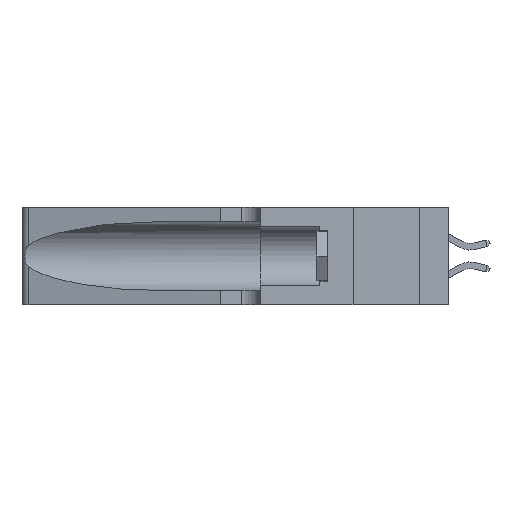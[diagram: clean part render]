
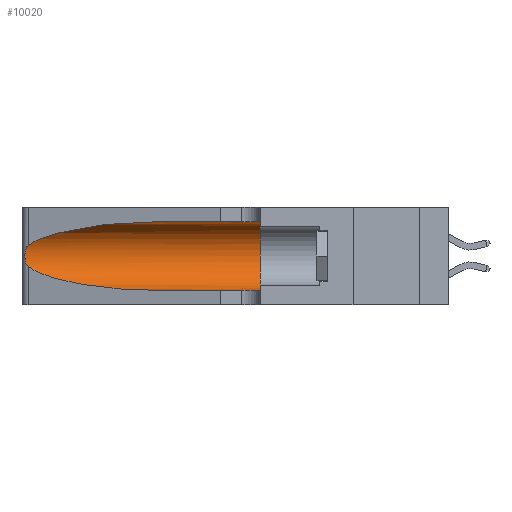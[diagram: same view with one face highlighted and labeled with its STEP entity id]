
A CAD part, left-side view. The second image highlights one B-rep face of the part: STEP entity #10020.
In plain terms, the highlighted cylindrical face has radius 3.308 mm (diameter 6.617 mm), a partial arc.
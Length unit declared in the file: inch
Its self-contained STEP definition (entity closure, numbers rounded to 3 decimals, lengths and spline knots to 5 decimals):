
#9 = CARTESIAN_POINT ( 'NONE',  ( 0.18966, 0.96281, 0.05475 ) ) ;
#45 = CARTESIAN_POINT ( 'NONE',  ( 0.25555, 1.22994, 0.2215 ) ) ;
#142 = LINE ( 'NONE', #4541, #23501 ) ;
#310 = CARTESIAN_POINT ( 'NONE',  ( 0.25555, 1.22993, 0.14849 ) ) ;
#469 = DIRECTION ( 'NONE',  ( 0., 0., 1. ) ) ;
#746 = EDGE_CURVE ( 'NONE', #12465, #10839, #22938, .T. ) ;
#1128 = DIRECTION ( 'NONE',  ( 0., -1., 0. ) ) ;
#1130 = DIRECTION ( 'NONE',  ( 0., -1., 0. ) ) ;
#1212 = DIRECTION ( 'NONE',  ( 0., 0., -1. ) ) ;
#1377 = CARTESIAN_POINT ( 'NONE',  ( 0.1305, 1.61858, 0.185 ) ) ;
#2003 = CARTESIAN_POINT ( 'NONE',  ( 0.26017, 1.23833, 0.17102 ) ) ;
#3063 = B_SPLINE_CURVE_WITH_KNOTS ( 'NONE', 3,
 ( #4125, #45, #13833, #4030, #6064, #17570, #15807, #13556, #2003, #5970, #15544, #9962, #310, #23531 ),
 .UNSPECIFIED., .F., .F.,
 ( 4, 2, 2, 2, 2, 2, 4 ),
 ( 0., 0.00027, 0.00053, 0.00107, 0.0016, 0.00187, 0.00214 ),
 .UNSPECIFIED. ) ;
#4030 = CARTESIAN_POINT ( 'NONE',  ( 0.25787, 1.23484, 0.2124 ) ) ;
#4125 = CARTESIAN_POINT ( 'NONE',  ( 0.25487, 1.22718, 0.22369 ) ) ;
#4434 = CARTESIAN_POINT ( 'NONE',  ( 0.1305, 0.35, 0.31525 ) ) ;
#4541 = CARTESIAN_POINT ( 'NONE',  ( 0.1305, 1.61858, 0.31525 ) ) ;
#4695 = LINE ( 'NONE', #10105, #17401 ) ;
#4782 = CYLINDRICAL_SURFACE ( 'NONE', #9889, 0.13025 ) ;
#4849 = CARTESIAN_POINT ( 'NONE',  ( 0.2373, 1.15595, 0.28018 ) ) ;
#5970 = CARTESIAN_POINT ( 'NONE',  ( 0.25856, 1.23593, 0.16098 ) ) ;
#6030 = CARTESIAN_POINT ( 'NONE',  ( 0.1305, 0.72297, 0.05475 ) ) ;
#6064 = CARTESIAN_POINT ( 'NONE',  ( 0.25854, 1.2359, 0.20912 ) ) ;
#6869 = EDGE_CURVE ( 'NONE', #24837, #12465, #3063, .T. ) ;
#6911 = ORIENTED_EDGE ( 'NONE', *, *, #746, .T. ) ;
#7009 = VERTEX_POINT ( 'NONE', #23465 ) ;
#7411 = VERTEX_POINT ( 'NONE', #11786 ) ;
#9354 = CIRCLE ( 'NONE', #14118, 0.13025 ) ;
#9669 = CARTESIAN_POINT ( 'NONE',  ( 0.2373, 1.15595, 0.08982 ) ) ;
#9889 = AXIS2_PLACEMENT_3D ( 'NONE', #1377, #1128, #1212 ) ;
#9962 = CARTESIAN_POINT ( 'NONE',  ( 0.25639, 1.23186, 0.15144 ) ) ;
#10020 = ADVANCED_FACE ( 'NONE', ( #11404 ), #4782, .F. ) ;
#10105 = CARTESIAN_POINT ( 'NONE',  ( 0.1305, 1.61858, 0.05475 ) ) ;
#10591 = CARTESIAN_POINT ( 'NONE',  ( 0.1305, 0.72297, 0.31525 ) ) ;
#10839 = VERTEX_POINT ( 'NONE', #24407 ) ;
#11404 = FACE_OUTER_BOUND ( 'NONE', #14740, .T. ) ;
#11680 = CARTESIAN_POINT ( 'NONE',  ( 0.25487, 1.22718, 0.14631 ) ) ;
#11786 = CARTESIAN_POINT ( 'NONE',  ( 0.1305, 0.72297, 0.31525 ) ) ;
#12046 = DIRECTION ( 'NONE',  ( 0., 1., 0. ) ) ;
#12465 = VERTEX_POINT ( 'NONE', #20478 ) ;
#12801 = ORIENTED_EDGE ( 'NONE', *, *, #19139, .F. ) ;
#12835 = EDGE_CURVE ( 'NONE', #21500, #7009, #9354, .T. ) ;
#13535 = CARTESIAN_POINT ( 'NONE',  ( 0.25487, 1.22718, 0.22369 ) ) ;
#13556 = CARTESIAN_POINT ( 'NONE',  ( 0.26075, 1.23896, 0.178 ) ) ;
#13833 = CARTESIAN_POINT ( 'NONE',  ( 0.25639, 1.23184, 0.21858 ) ) ;
#14118 = AXIS2_PLACEMENT_3D ( 'NONE', #23687, #12046, #469 ) ;
#14135 = ORIENTED_EDGE ( 'NONE', *, *, #16243, .T. ) ;
#14483 = CARTESIAN_POINT ( 'NONE',  ( 0.18966, 0.96281, 0.31525 ) ) ;
#14740 = EDGE_LOOP ( 'NONE', ( #18365, #14761, #6911, #14135, #16877, #12801 ) ) ;
#14761 = ORIENTED_EDGE ( 'NONE', *, *, #6869, .T. ) ;
#15544 = CARTESIAN_POINT ( 'NONE',  ( 0.25789, 1.23486, 0.15765 ) ) ;
#15807 = CARTESIAN_POINT ( 'NONE',  ( 0.26075, 1.23896, 0.19203 ) ) ;
#16243 = EDGE_CURVE ( 'NONE', #10839, #7009, #4695, .T. ) ;
#16877 = ORIENTED_EDGE ( 'NONE', *, *, #12835, .F. ) ;
#17401 = VECTOR ( 'NONE', #21383, 39.37008 ) ;
#17570 = CARTESIAN_POINT ( 'NONE',  ( 0.26018, 1.23835, 0.19895 ) ) ;
#17954 = EDGE_CURVE ( 'NONE', #7411, #24837, #19097, .T. ) ;
#18365 = ORIENTED_EDGE ( 'NONE', *, *, #17954, .T. ) ;
#18400 = CARTESIAN_POINT ( 'NONE',  ( 0.25487, 1.22718, 0.22369 ) ) ;
#19097 =( BOUNDED_CURVE ( )  B_SPLINE_CURVE ( 3, ( #10591, #14483, #4849, #18400 ),
 .UNSPECIFIED., .F., .T. ) 
 B_SPLINE_CURVE_WITH_KNOTS ( ( 4, 4 ),
 ( 1.5708, 2.84003 ),
 .UNSPECIFIED. ) 
 CURVE ( )  GEOMETRIC_REPRESENTATION_ITEM ( )  RATIONAL_B_SPLINE_CURVE ( ( 1., 0.87, 0.87, 1. ) ) 
 REPRESENTATION_ITEM ( '' )  );
#19139 = EDGE_CURVE ( 'NONE', #7411, #21500, #142, .T. ) ;
#20478 = CARTESIAN_POINT ( 'NONE',  ( 0.25487, 1.22718, 0.14631 ) ) ;
#21383 = DIRECTION ( 'NONE',  ( 0., -1., 0. ) ) ;
#21500 = VERTEX_POINT ( 'NONE', #4434 ) ;
#22938 =( BOUNDED_CURVE ( )  B_SPLINE_CURVE ( 3, ( #11680, #9669, #9, #6030 ),
 .UNSPECIFIED., .F., .T. ) 
 B_SPLINE_CURVE_WITH_KNOTS ( ( 4, 4 ),
 ( 3.44316, 4.71239 ),
 .UNSPECIFIED. ) 
 CURVE ( )  GEOMETRIC_REPRESENTATION_ITEM ( )  RATIONAL_B_SPLINE_CURVE ( ( 1., 0.87, 0.87, 1. ) ) 
 REPRESENTATION_ITEM ( '' )  );
#23465 = CARTESIAN_POINT ( 'NONE',  ( 0.1305, 0.35, 0.05475 ) ) ;
#23501 = VECTOR ( 'NONE', #1130, 39.37008 ) ;
#23531 = CARTESIAN_POINT ( 'NONE',  ( 0.25487, 1.22718, 0.14631 ) ) ;
#23687 = CARTESIAN_POINT ( 'NONE',  ( 0.1305, 0.35, 0.185 ) ) ;
#24407 = CARTESIAN_POINT ( 'NONE',  ( 0.1305, 0.72297, 0.05475 ) ) ;
#24837 = VERTEX_POINT ( 'NONE', #13535 ) ;
